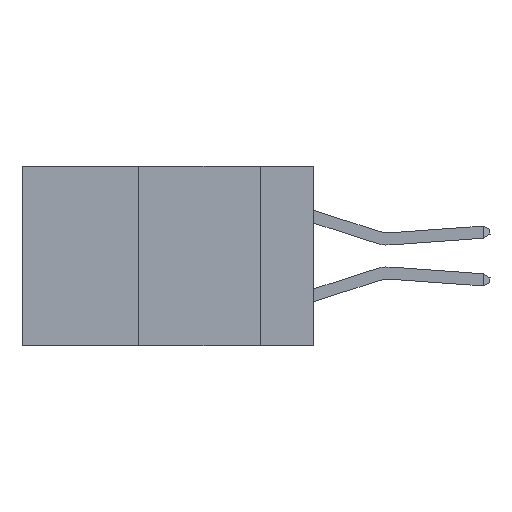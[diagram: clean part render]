
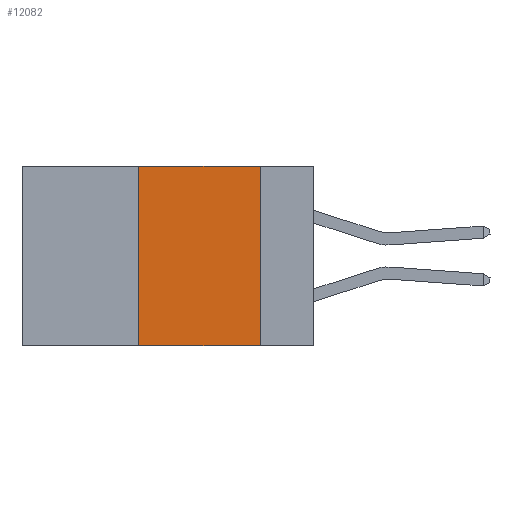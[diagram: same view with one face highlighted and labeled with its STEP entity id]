
A CAD part, left-side view. The second image highlights one B-rep face of the part: STEP entity #12082.
In plain terms, the highlighted planar face has unit normal (-1, 0, 0).
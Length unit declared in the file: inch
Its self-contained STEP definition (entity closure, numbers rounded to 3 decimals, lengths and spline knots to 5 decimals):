
#1966 = CARTESIAN_POINT ( 'NONE',  ( 0., 0.6, 0. ) ) ;
#2497 = CARTESIAN_POINT ( 'NONE',  ( 0., 0.36, -0.37 ) ) ;
#2849 = VERTEX_POINT ( 'NONE', #11115 ) ;
#3431 = EDGE_CURVE ( 'NONE', #4674, #21821, #18022, .T. ) ;
#3731 = LINE ( 'NONE', #8846, #18535 ) ;
#3861 = DIRECTION ( 'NONE',  ( 0., -1., 0. ) ) ;
#4674 = VERTEX_POINT ( 'NONE', #22156 ) ;
#5287 = CARTESIAN_POINT ( 'NONE',  ( 0., 0.6, 0. ) ) ;
#5400 = ORIENTED_EDGE ( 'NONE', *, *, #5804, .F. ) ;
#5804 = EDGE_CURVE ( 'NONE', #21821, #2849, #3731, .T. ) ;
#5831 = EDGE_LOOP ( 'NONE', ( #5400, #15282, #6016, #10930 ) ) ;
#6016 = ORIENTED_EDGE ( 'NONE', *, *, #8297, .F. ) ;
#7193 = DIRECTION ( 'NONE',  ( 0., 0., -1. ) ) ;
#7980 = VECTOR ( 'NONE', #15965, 39.37008 ) ;
#8297 = EDGE_CURVE ( 'NONE', #20820, #4674, #13258, .T. ) ;
#8520 = CARTESIAN_POINT ( 'NONE',  ( 0., 0.6, -0.37 ) ) ;
#8846 = CARTESIAN_POINT ( 'NONE',  ( 0., 0.11, 0. ) ) ;
#8888 = VECTOR ( 'NONE', #18875, 39.37008 ) ;
#10930 = ORIENTED_EDGE ( 'NONE', *, *, #14187, .T. ) ;
#11115 = CARTESIAN_POINT ( 'NONE',  ( 0., 0.11, -0.37 ) ) ;
#11125 = CARTESIAN_POINT ( 'NONE',  ( 0., 0.11, 0. ) ) ;
#12082 = ADVANCED_FACE ( 'NONE', ( #14119 ), #16389, .F. ) ;
#13171 = VECTOR ( 'NONE', #3861, 39.37008 ) ;
#13258 = LINE ( 'NONE', #22560, #8888 ) ;
#14119 = FACE_OUTER_BOUND ( 'NONE', #5831, .T. ) ;
#14187 = EDGE_CURVE ( 'NONE', #20820, #2849, #22657, .T. ) ;
#15282 = ORIENTED_EDGE ( 'NONE', *, *, #3431, .F. ) ;
#15965 = DIRECTION ( 'NONE',  ( 0., -1., 0. ) ) ;
#16389 = PLANE ( 'NONE',  #16946 ) ;
#16946 = AXIS2_PLACEMENT_3D ( 'NONE', #5287, #18235, #7193 ) ;
#18022 = LINE ( 'NONE', #1966, #13171 ) ;
#18235 = DIRECTION ( 'NONE',  ( 1., 0., 0. ) ) ;
#18535 = VECTOR ( 'NONE', #21719, 39.37008 ) ;
#18875 = DIRECTION ( 'NONE',  ( 0., 0., 1. ) ) ;
#20820 = VERTEX_POINT ( 'NONE', #2497 ) ;
#21719 = DIRECTION ( 'NONE',  ( 0., 0., -1. ) ) ;
#21821 = VERTEX_POINT ( 'NONE', #11125 ) ;
#22156 = CARTESIAN_POINT ( 'NONE',  ( 0., 0.36, 0. ) ) ;
#22560 = CARTESIAN_POINT ( 'NONE',  ( 0., 0.36, 0. ) ) ;
#22657 = LINE ( 'NONE', #8520, #7980 ) ;
